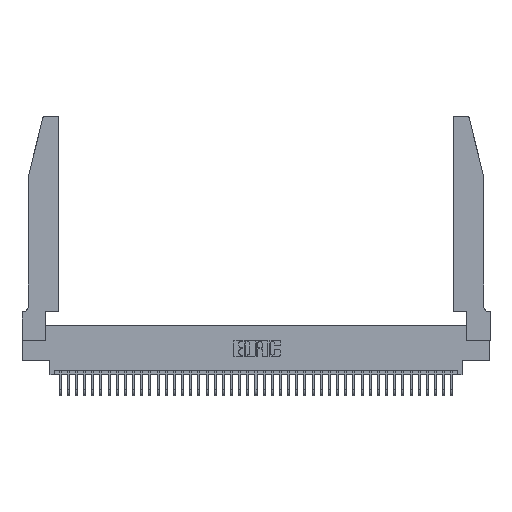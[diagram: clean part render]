
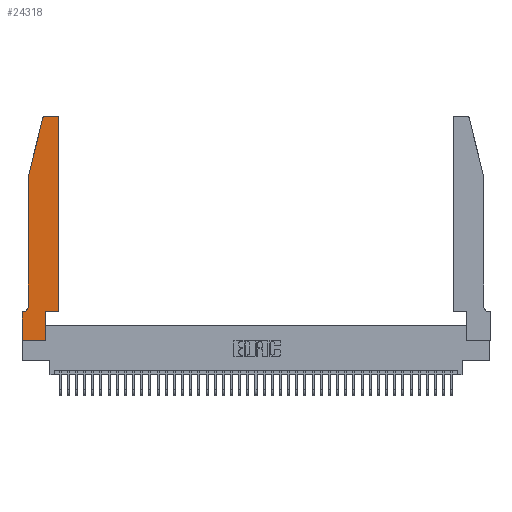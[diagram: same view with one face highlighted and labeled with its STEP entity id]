
A CAD part, top view. The second image highlights one B-rep face of the part: STEP entity #24318.
In plain terms, the highlighted planar face has unit normal (0, 0, 1).
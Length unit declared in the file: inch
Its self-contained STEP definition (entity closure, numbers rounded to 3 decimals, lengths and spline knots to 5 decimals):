
#155 = CARTESIAN_POINT ( 'NONE',  ( 0.0055, 0.42, 0.37 ) ) ;
#882 = CARTESIAN_POINT ( 'NONE',  ( 0.4205, 2.72, 0.37 ) ) ;
#885 = EDGE_CURVE ( 'NONE', #21387, #33550, #18740, .T. ) ;
#1147 = VERTEX_POINT ( 'NONE', #2649 ) ;
#1660 = LINE ( 'NONE', #24129, #40647 ) ;
#1773 = DIRECTION ( 'NONE',  ( 0., -1., 0. ) ) ;
#2023 = CARTESIAN_POINT ( 'NONE',  ( 0.2865, 0., 0.37 ) ) ;
#2579 = EDGE_CURVE ( 'NONE', #9317, #29593, #14746, .T. ) ;
#2649 = CARTESIAN_POINT ( 'NONE',  ( 0.284, 2.75, 0.37 ) ) ;
#2665 = CARTESIAN_POINT ( 'NONE',  ( 0., 0.35, 0.37 ) ) ;
#3285 = VECTOR ( 'NONE', #15806, 39.37008 ) ;
#3327 = DIRECTION ( 'NONE',  ( -1., 0., 0. ) ) ;
#3775 = CARTESIAN_POINT ( 'NONE',  ( 0., 0.35, 0.37 ) ) ;
#4068 = DIRECTION ( 'NONE',  ( 1., 0., 0. ) ) ;
#4342 = VECTOR ( 'NONE', #15749, 39.37008 ) ;
#4375 = VERTEX_POINT ( 'NONE', #34229 ) ;
#4896 = CIRCLE ( 'NONE', #11724, 0.03 ) ;
#5250 = EDGE_LOOP ( 'NONE', ( #40773, #37852, #32442, #7787, #26538, #36869, #23103, #21600, #24571, #22120, #16742, #7856 ) ) ;
#5876 = DIRECTION ( 'NONE',  ( 1., 0., 0. ) ) ;
#7352 = CARTESIAN_POINT ( 'NONE',  ( 0.0055, 0.35, 0.37 ) ) ;
#7787 = ORIENTED_EDGE ( 'NONE', *, *, #20443, .T. ) ;
#7856 = ORIENTED_EDGE ( 'NONE', *, *, #885, .T. ) ;
#8396 = DIRECTION ( 'NONE',  ( 0., 1., 0. ) ) ;
#9317 = VERTEX_POINT ( 'NONE', #13311 ) ;
#10134 = VERTEX_POINT ( 'NONE', #27818 ) ;
#10473 = LINE ( 'NONE', #13618, #25252 ) ;
#11720 = LINE ( 'NONE', #31523, #3285 ) ;
#11724 = AXIS2_PLACEMENT_3D ( 'NONE', #31057, #12172, #34242 ) ;
#12172 = DIRECTION ( 'NONE',  ( 0., 0., 1. ) ) ;
#12876 = VERTEX_POINT ( 'NONE', #7352 ) ;
#13311 = CARTESIAN_POINT ( 'NONE',  ( 0.25487, 2.72718, 0.37 ) ) ;
#13618 = CARTESIAN_POINT ( 'NONE',  ( 0.0755, 2., 0.37 ) ) ;
#13751 = DIRECTION ( 'NONE',  ( 0., -1., 0. ) ) ;
#14746 = LINE ( 'NONE', #31464, #4342 ) ;
#15749 = DIRECTION ( 'NONE',  ( -0.239, -0.971, 0. ) ) ;
#15806 = DIRECTION ( 'NONE',  ( -1., 0., 0. ) ) ;
#15877 = AXIS2_PLACEMENT_3D ( 'NONE', #155, #22242, #3327 ) ;
#16742 = ORIENTED_EDGE ( 'NONE', *, *, #29742, .T. ) ;
#18416 = CARTESIAN_POINT ( 'NONE',  ( 0.4505, 0.35, 0.37 ) ) ;
#18645 = CIRCLE ( 'NONE', #15877, 0.07 ) ;
#18740 = CIRCLE ( 'NONE', #30040, 0.03 ) ;
#19349 = EDGE_CURVE ( 'NONE', #38864, #10134, #1660, .T. ) ;
#19512 = VECTOR ( 'NONE', #21573, 39.37008 ) ;
#19719 = CARTESIAN_POINT ( 'NONE',  ( 0.4205, 2.75, 0.37 ) ) ;
#19945 = DIRECTION ( 'NONE',  ( -1., 0., 0. ) ) ;
#20443 = EDGE_CURVE ( 'NONE', #29593, #29390, #10473, .T. ) ;
#20806 = VECTOR ( 'NONE', #19945, 39.37008 ) ;
#20900 = CARTESIAN_POINT ( 'NONE',  ( 0.0755, 2., 0.37 ) ) ;
#21387 = VERTEX_POINT ( 'NONE', #34485 ) ;
#21573 = DIRECTION ( 'NONE',  ( 0., 1., 0. ) ) ;
#21600 = ORIENTED_EDGE ( 'NONE', *, *, #25383, .T. ) ;
#22120 = ORIENTED_EDGE ( 'NONE', *, *, #26507, .T. ) ;
#22242 = DIRECTION ( 'NONE',  ( 0., 0., -1. ) ) ;
#22997 = DIRECTION ( 'NONE',  ( 0., 0., 1. ) ) ;
#23103 = ORIENTED_EDGE ( 'NONE', *, *, #26990, .T. ) ;
#23265 = LINE ( 'NONE', #30073, #39049 ) ;
#24129 = CARTESIAN_POINT ( 'NONE',  ( 0.2865, 0.35, 0.37 ) ) ;
#24258 = VECTOR ( 'NONE', #37416, 39.37008 ) ;
#24318 = ADVANCED_FACE ( 'NONE', ( #40674 ), #37336, .T. ) ;
#24571 = ORIENTED_EDGE ( 'NONE', *, *, #19349, .T. ) ;
#24758 = DIRECTION ( 'NONE',  ( 0., 0., 1. ) ) ;
#25247 = LINE ( 'NONE', #40578, #24258 ) ;
#25252 = VECTOR ( 'NONE', #13751, 39.37008 ) ;
#25275 = VECTOR ( 'NONE', #34201, 39.37008 ) ;
#25383 = EDGE_CURVE ( 'NONE', #25863, #38864, #34688, .T. ) ;
#25685 = EDGE_CURVE ( 'NONE', #33550, #1147, #30193, .T. ) ;
#25863 = VERTEX_POINT ( 'NONE', #39548 ) ;
#26507 = EDGE_CURVE ( 'NONE', #10134, #4375, #25247, .T. ) ;
#26538 = ORIENTED_EDGE ( 'NONE', *, *, #34661, .T. ) ;
#26990 = EDGE_CURVE ( 'NONE', #36107, #25863, #23265, .T. ) ;
#27818 = CARTESIAN_POINT ( 'NONE',  ( 0.2865, 0.35, 0.37 ) ) ;
#29347 = CARTESIAN_POINT ( 'NONE',  ( 0.0755, 0.42, 0.37 ) ) ;
#29390 = VERTEX_POINT ( 'NONE', #29347 ) ;
#29593 = VERTEX_POINT ( 'NONE', #20900 ) ;
#29662 = AXIS2_PLACEMENT_3D ( 'NONE', #2665, #24758, #5876 ) ;
#29742 = EDGE_CURVE ( 'NONE', #4375, #21387, #36342, .T. ) ;
#30040 = AXIS2_PLACEMENT_3D ( 'NONE', #882, #22997, #4068 ) ;
#30073 = CARTESIAN_POINT ( 'NONE',  ( 0., 0., 0.37 ) ) ;
#30193 = LINE ( 'NONE', #35713, #20806 ) ;
#31057 = CARTESIAN_POINT ( 'NONE',  ( 0.284, 2.72, 0.37 ) ) ;
#31464 = CARTESIAN_POINT ( 'NONE',  ( 0.0755, 2., 0.37 ) ) ;
#31523 = CARTESIAN_POINT ( 'NONE',  ( 0.0755, 0.35, 0.37 ) ) ;
#32442 = ORIENTED_EDGE ( 'NONE', *, *, #2579, .T. ) ;
#33550 = VERTEX_POINT ( 'NONE', #19719 ) ;
#34201 = DIRECTION ( 'NONE',  ( 1., 0., 0. ) ) ;
#34229 = CARTESIAN_POINT ( 'NONE',  ( 0.4505, 0.35, 0.37 ) ) ;
#34242 = DIRECTION ( 'NONE',  ( 1., 0., 0. ) ) ;
#34485 = CARTESIAN_POINT ( 'NONE',  ( 0.4505, 2.72, 0.37 ) ) ;
#34661 = EDGE_CURVE ( 'NONE', #29390, #12876, #18645, .T. ) ;
#34688 = LINE ( 'NONE', #40518, #25275 ) ;
#35713 = CARTESIAN_POINT ( 'NONE',  ( 0.2605, 2.75, 0.37 ) ) ;
#36107 = VERTEX_POINT ( 'NONE', #3775 ) ;
#36342 = LINE ( 'NONE', #18416, #19512 ) ;
#36869 = ORIENTED_EDGE ( 'NONE', *, *, #39479, .T. ) ;
#37336 = PLANE ( 'NONE',  #29662 ) ;
#37416 = DIRECTION ( 'NONE',  ( 1., 0., 0. ) ) ;
#37852 = ORIENTED_EDGE ( 'NONE', *, *, #38324, .T. ) ;
#38324 = EDGE_CURVE ( 'NONE', #1147, #9317, #4896, .T. ) ;
#38864 = VERTEX_POINT ( 'NONE', #2023 ) ;
#39049 = VECTOR ( 'NONE', #1773, 39.37008 ) ;
#39479 = EDGE_CURVE ( 'NONE', #12876, #36107, #11720, .T. ) ;
#39548 = CARTESIAN_POINT ( 'NONE',  ( 0., 0., 0.37 ) ) ;
#40518 = CARTESIAN_POINT ( 'NONE',  ( 0., 0., 0.37 ) ) ;
#40578 = CARTESIAN_POINT ( 'NONE',  ( 0.4505, 0.35, 0.37 ) ) ;
#40647 = VECTOR ( 'NONE', #8396, 39.37008 ) ;
#40674 = FACE_OUTER_BOUND ( 'NONE', #5250, .T. ) ;
#40773 = ORIENTED_EDGE ( 'NONE', *, *, #25685, .T. ) ;
